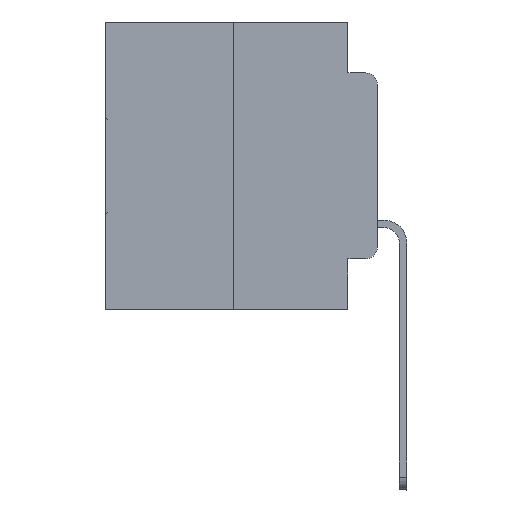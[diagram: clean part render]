
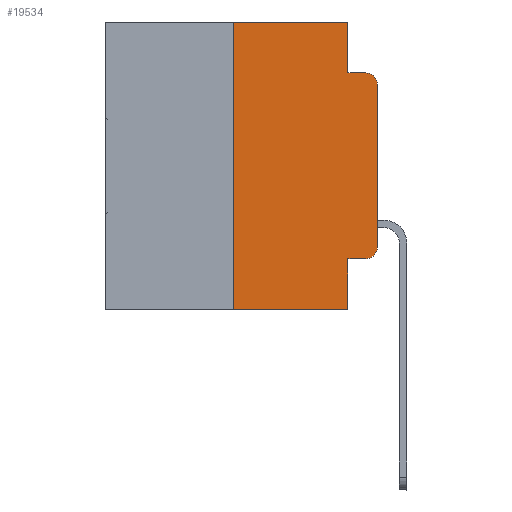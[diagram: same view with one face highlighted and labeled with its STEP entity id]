
A CAD part, left-side view. The second image highlights one B-rep face of the part: STEP entity #19534.
In plain terms, the highlighted planar face has unit normal (-1, 0, 0).
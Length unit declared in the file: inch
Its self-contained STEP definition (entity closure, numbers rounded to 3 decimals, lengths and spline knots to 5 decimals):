
#393 = DIRECTION ( 'NONE',  ( 0., 0., -1. ) ) ;
#1042 = CARTESIAN_POINT ( 'NONE',  ( 0., 0.051, 0. ) ) ;
#1213 = CARTESIAN_POINT ( 'NONE',  ( 0., 0.051, -0.4115 ) ) ;
#1713 = VERTEX_POINT ( 'NONE', #21251 ) ;
#1767 = ORIENTED_EDGE ( 'NONE', *, *, #2200, .F. ) ;
#1882 = EDGE_CURVE ( 'NONE', #22502, #25581, #22609, .T. ) ;
#2200 = EDGE_CURVE ( 'NONE', #18787, #1713, #8062, .T. ) ;
#2556 = CARTESIAN_POINT ( 'NONE',  ( 0., 0.473, 0. ) ) ;
#2559 = ORIENTED_EDGE ( 'NONE', *, *, #24605, .T. ) ;
#2811 = ORIENTED_EDGE ( 'NONE', *, *, #1882, .T. ) ;
#3479 = DIRECTION ( 'NONE',  ( 0., 0., -1. ) ) ;
#3658 = CARTESIAN_POINT ( 'NONE',  ( 0., 0.25, 0. ) ) ;
#3751 = AXIS2_PLACEMENT_3D ( 'NONE', #23579, #28336, #7227 ) ;
#5245 = ORIENTED_EDGE ( 'NONE', *, *, #10651, .T. ) ;
#5412 = AXIS2_PLACEMENT_3D ( 'NONE', #2556, #16912, #393 ) ;
#5619 = EDGE_CURVE ( 'NONE', #19898, #5847, #27665, .T. ) ;
#5789 = LINE ( 'NONE', #1042, #20466 ) ;
#5847 = VERTEX_POINT ( 'NONE', #29069 ) ;
#6435 = VECTOR ( 'NONE', #13043, 39.37008 ) ;
#6542 = FACE_OUTER_BOUND ( 'NONE', #8634, .T. ) ;
#6826 = DIRECTION ( 'NONE',  ( 0., -1., 0. ) ) ;
#7227 = DIRECTION ( 'NONE',  ( 0., 0., -1. ) ) ;
#7243 = VERTEX_POINT ( 'NONE', #27608 ) ;
#7983 = VECTOR ( 'NONE', #3479, 39.37008 ) ;
#8032 = VECTOR ( 'NONE', #19875, 39.37008 ) ;
#8062 = LINE ( 'NONE', #24252, #7983 ) ;
#8416 = CARTESIAN_POINT ( 'NONE',  ( 0., 0.051, 0. ) ) ;
#8634 = EDGE_LOOP ( 'NONE', ( #9656, #5245, #27241, #1767, #17463, #14645, #2811, #19199, #2559, #25596 ) ) ;
#9428 = LINE ( 'NONE', #23335, #27490 ) ;
#9656 = ORIENTED_EDGE ( 'NONE', *, *, #12006, .T. ) ;
#10651 = EDGE_CURVE ( 'NONE', #7243, #29888, #20049, .T. ) ;
#11034 = CARTESIAN_POINT ( 'NONE',  ( 0., 0.02, -0.1085 ) ) ;
#11042 = CARTESIAN_POINT ( 'NONE',  ( 0., 0.051, -0.5 ) ) ;
#12006 = EDGE_CURVE ( 'NONE', #5847, #7243, #22782, .T. ) ;
#12910 = EDGE_CURVE ( 'NONE', #21739, #18787, #29911, .T. ) ;
#13043 = DIRECTION ( 'NONE',  ( 0., 0., 1. ) ) ;
#13408 = EDGE_CURVE ( 'NONE', #22502, #21739, #24673, .T. ) ;
#13916 = CARTESIAN_POINT ( 'NONE',  ( 0., 0., 0. ) ) ;
#14243 = VECTOR ( 'NONE', #22950, 39.37008 ) ;
#14645 = ORIENTED_EDGE ( 'NONE', *, *, #13408, .F. ) ;
#15949 = CARTESIAN_POINT ( 'NONE',  ( 0., 0.25, 0. ) ) ;
#16426 = EDGE_CURVE ( 'NONE', #24698, #25581, #5789, .T. ) ;
#16912 = DIRECTION ( 'NONE',  ( 1., 0., 0. ) ) ;
#17463 = ORIENTED_EDGE ( 'NONE', *, *, #12910, .F. ) ;
#17624 = DIRECTION ( 'NONE',  ( 0., 0., -1. ) ) ;
#18737 = CARTESIAN_POINT ( 'NONE',  ( 0., 0.25, -0.5 ) ) ;
#18787 = VERTEX_POINT ( 'NONE', #8416 ) ;
#19199 = ORIENTED_EDGE ( 'NONE', *, *, #16426, .F. ) ;
#19534 = ADVANCED_FACE ( 'NONE', ( #6542 ), #27934, .F. ) ;
#19875 = DIRECTION ( 'NONE',  ( 0., -1., 0. ) ) ;
#19898 = VERTEX_POINT ( 'NONE', #23126 ) ;
#20049 = CIRCLE ( 'NONE', #23001, 0.02 ) ;
#20466 = VECTOR ( 'NONE', #29182, 39.37008 ) ;
#21251 = CARTESIAN_POINT ( 'NONE',  ( 0., 0.051, -0.0885 ) ) ;
#21739 = VERTEX_POINT ( 'NONE', #3658 ) ;
#22502 = VERTEX_POINT ( 'NONE', #18737 ) ;
#22609 = LINE ( 'NONE', #24451, #26624 ) ;
#22624 = CARTESIAN_POINT ( 'NONE',  ( 0., 0.051, -0.4115 ) ) ;
#22782 = LINE ( 'NONE', #13916, #14243 ) ;
#22950 = DIRECTION ( 'NONE',  ( 0., 0., 1. ) ) ;
#23001 = AXIS2_PLACEMENT_3D ( 'NONE', #11034, #27243, #17624 ) ;
#23126 = CARTESIAN_POINT ( 'NONE',  ( 0., 0.02, -0.4115 ) ) ;
#23335 = CARTESIAN_POINT ( 'NONE',  ( 0., 0.051, -0.0885 ) ) ;
#23537 = EDGE_CURVE ( 'NONE', #1713, #29888, #9428, .T. ) ;
#23579 = CARTESIAN_POINT ( 'NONE',  ( 0., 0.02, -0.3915 ) ) ;
#24026 = CARTESIAN_POINT ( 'NONE',  ( 0., 0.02, -0.0885 ) ) ;
#24252 = CARTESIAN_POINT ( 'NONE',  ( 0., 0.051, 0. ) ) ;
#24451 = CARTESIAN_POINT ( 'NONE',  ( 0., 0.473, -0.5 ) ) ;
#24605 = EDGE_CURVE ( 'NONE', #24698, #19898, #26917, .T. ) ;
#24673 = LINE ( 'NONE', #15949, #6435 ) ;
#24698 = VERTEX_POINT ( 'NONE', #22624 ) ;
#25581 = VERTEX_POINT ( 'NONE', #11042 ) ;
#25596 = ORIENTED_EDGE ( 'NONE', *, *, #5619, .T. ) ;
#25945 = VECTOR ( 'NONE', #6826, 39.37008 ) ;
#26624 = VECTOR ( 'NONE', #29495, 39.37008 ) ;
#26917 = LINE ( 'NONE', #1213, #8032 ) ;
#27241 = ORIENTED_EDGE ( 'NONE', *, *, #23537, .F. ) ;
#27243 = DIRECTION ( 'NONE',  ( -1., 0., 0. ) ) ;
#27490 = VECTOR ( 'NONE', #27771, 39.37008 ) ;
#27608 = CARTESIAN_POINT ( 'NONE',  ( 0., 0., -0.1085 ) ) ;
#27665 = CIRCLE ( 'NONE', #3751, 0.02 ) ;
#27771 = DIRECTION ( 'NONE',  ( 0., -1., 0. ) ) ;
#27934 = PLANE ( 'NONE',  #5412 ) ;
#28336 = DIRECTION ( 'NONE',  ( -1., 0., 0. ) ) ;
#29069 = CARTESIAN_POINT ( 'NONE',  ( 0., 0., -0.3915 ) ) ;
#29182 = DIRECTION ( 'NONE',  ( 0., 0., -1. ) ) ;
#29495 = DIRECTION ( 'NONE',  ( 0., -1., 0. ) ) ;
#29598 = CARTESIAN_POINT ( 'NONE',  ( 0., 0.473, 0. ) ) ;
#29888 = VERTEX_POINT ( 'NONE', #24026 ) ;
#29911 = LINE ( 'NONE', #29598, #25945 ) ;
